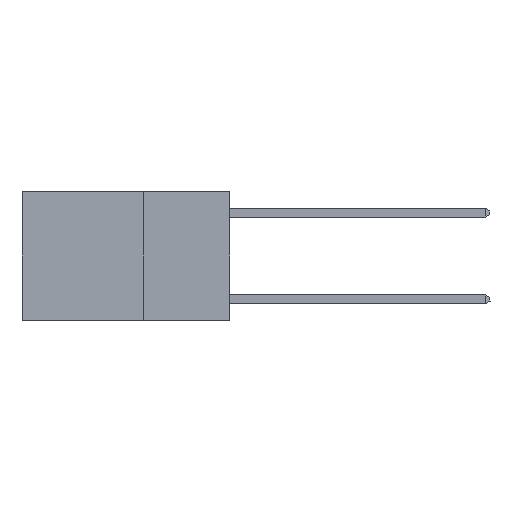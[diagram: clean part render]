
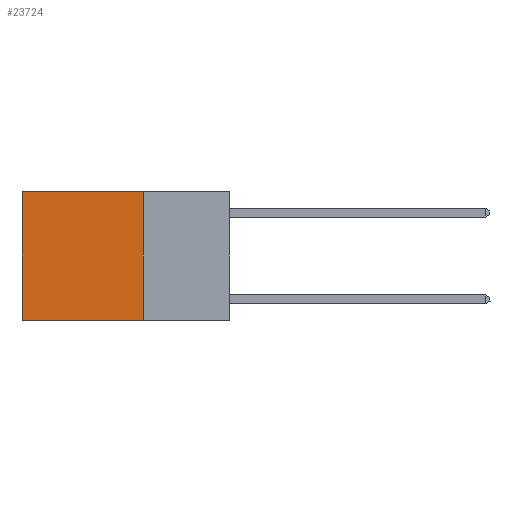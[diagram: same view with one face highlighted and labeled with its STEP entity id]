
A CAD part, left-side view. The second image highlights one B-rep face of the part: STEP entity #23724.
In plain terms, the highlighted planar face has unit normal (-1, 0, 0).
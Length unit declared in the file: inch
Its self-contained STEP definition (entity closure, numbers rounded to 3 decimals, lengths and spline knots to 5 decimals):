
#271 = VECTOR ( 'NONE', #12719, 39.37008 ) ;
#1901 = AXIS2_PLACEMENT_3D ( 'NONE', #22543, #7612, #25057 ) ;
#2537 = LINE ( 'NONE', #8729, #21726 ) ;
#3775 = ORIENTED_EDGE ( 'NONE', *, *, #10953, .T. ) ;
#3886 = ORIENTED_EDGE ( 'NONE', *, *, #29839, .F. ) ;
#4385 = CARTESIAN_POINT ( 'NONE',  ( 0.2625, 0.25, 0. ) ) ;
#5082 = PLANE ( 'NONE',  #1901 ) ;
#5533 = VECTOR ( 'NONE', #31454, 39.37008 ) ;
#6112 = ORIENTED_EDGE ( 'NONE', *, *, #12966, .T. ) ;
#6188 = DIRECTION ( 'NONE',  ( 0., 1., 0. ) ) ;
#6951 = LINE ( 'NONE', #7538, #271 ) ;
#7538 = CARTESIAN_POINT ( 'NONE',  ( 0.2625, 0.25, -0.37 ) ) ;
#7612 = DIRECTION ( 'NONE',  ( 1., 0., 0. ) ) ;
#8724 = LINE ( 'NONE', #18344, #27781 ) ;
#8729 = CARTESIAN_POINT ( 'NONE',  ( 0.2625, 0.25, 0. ) ) ;
#10953 = EDGE_CURVE ( 'NONE', #28515, #14225, #2537, .T. ) ;
#12719 = DIRECTION ( 'NONE',  ( 0., 1., 0. ) ) ;
#12966 = EDGE_CURVE ( 'NONE', #14225, #27704, #19662, .T. ) ;
#14216 = CARTESIAN_POINT ( 'NONE',  ( 0.2625, 0.6, -0.37 ) ) ;
#14225 = VERTEX_POINT ( 'NONE', #23789 ) ;
#15753 = VERTEX_POINT ( 'NONE', #19284 ) ;
#18344 = CARTESIAN_POINT ( 'NONE',  ( 0.2625, 0.25, 0. ) ) ;
#19051 = FACE_OUTER_BOUND ( 'NONE', #22718, .T. ) ;
#19284 = CARTESIAN_POINT ( 'NONE',  ( 0.2625, 0.25, -0.37 ) ) ;
#19662 = LINE ( 'NONE', #26485, #5533 ) ;
#20834 = DIRECTION ( 'NONE',  ( 0., 0., -1. ) ) ;
#21726 = VECTOR ( 'NONE', #6188, 39.37008 ) ;
#22543 = CARTESIAN_POINT ( 'NONE',  ( 0.2625, 0.25, 0. ) ) ;
#22718 = EDGE_LOOP ( 'NONE', ( #6112, #26188, #3886, #3775 ) ) ;
#23038 = EDGE_CURVE ( 'NONE', #15753, #27704, #6951, .T. ) ;
#23724 = ADVANCED_FACE ( 'NONE', ( #19051 ), #5082, .F. ) ;
#23789 = CARTESIAN_POINT ( 'NONE',  ( 0.2625, 0.6, 0. ) ) ;
#25057 = DIRECTION ( 'NONE',  ( 0., 0., -1. ) ) ;
#26188 = ORIENTED_EDGE ( 'NONE', *, *, #23038, .F. ) ;
#26485 = CARTESIAN_POINT ( 'NONE',  ( 0.2625, 0.6, 0. ) ) ;
#27704 = VERTEX_POINT ( 'NONE', #14216 ) ;
#27781 = VECTOR ( 'NONE', #20834, 39.37008 ) ;
#28515 = VERTEX_POINT ( 'NONE', #4385 ) ;
#29839 = EDGE_CURVE ( 'NONE', #28515, #15753, #8724, .T. ) ;
#31454 = DIRECTION ( 'NONE',  ( 0., 0., -1. ) ) ;
